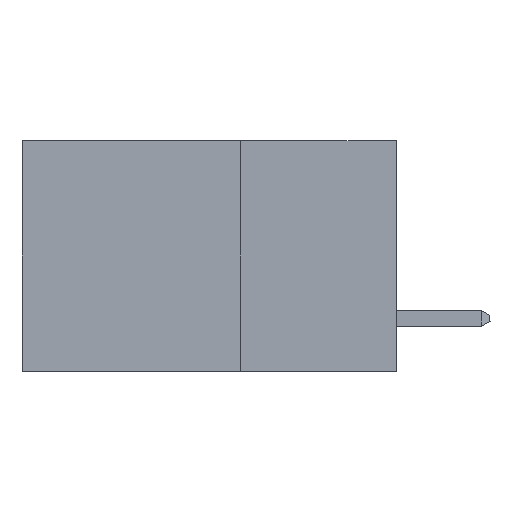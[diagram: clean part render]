
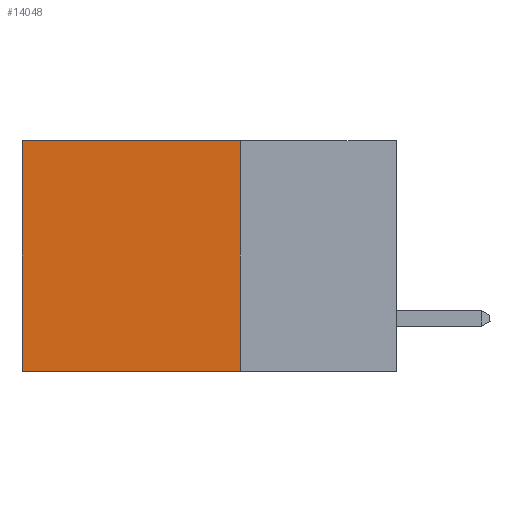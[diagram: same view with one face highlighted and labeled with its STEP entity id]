
A CAD part, left-side view. The second image highlights one B-rep face of the part: STEP entity #14048.
In plain terms, the highlighted planar face has unit normal (-1, 0, 0).
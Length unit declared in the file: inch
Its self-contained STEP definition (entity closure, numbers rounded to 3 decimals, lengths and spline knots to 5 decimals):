
#920 = DIRECTION ( 'NONE',  ( 0., 0., -1. ) ) ;
#1047 = DIRECTION ( 'NONE',  ( 0., 0., -1. ) ) ;
#1965 = VERTEX_POINT ( 'NONE', #13545 ) ;
#2149 = EDGE_LOOP ( 'NONE', ( #12952, #14968, #3069, #15810 ) ) ;
#2204 = FACE_OUTER_BOUND ( 'NONE', #2149, .T. ) ;
#2735 = LINE ( 'NONE', #10248, #9477 ) ;
#3069 = ORIENTED_EDGE ( 'NONE', *, *, #10551, .F. ) ;
#4941 = CARTESIAN_POINT ( 'NONE',  ( 0.298, 0.6, 0. ) ) ;
#5247 = DIRECTION ( 'NONE',  ( 0., 1., 0. ) ) ;
#5444 = EDGE_CURVE ( 'NONE', #1965, #18133, #12500, .T. ) ;
#5605 = CARTESIAN_POINT ( 'NONE',  ( 0.298, 0.6, -0.37 ) ) ;
#7328 = CARTESIAN_POINT ( 'NONE',  ( 0.298, 0.6, 0. ) ) ;
#7790 = DIRECTION ( 'NONE',  ( 1., 0., 0. ) ) ;
#9372 = DIRECTION ( 'NONE',  ( 0., 0., -1. ) ) ;
#9477 = VECTOR ( 'NONE', #5247, 39.37008 ) ;
#9799 = EDGE_CURVE ( 'NONE', #13871, #17910, #2735, .T. ) ;
#10248 = CARTESIAN_POINT ( 'NONE',  ( 0.298, 0.25, 0. ) ) ;
#10551 = EDGE_CURVE ( 'NONE', #13871, #1965, #19271, .T. ) ;
#12500 = LINE ( 'NONE', #14254, #20252 ) ;
#12952 = ORIENTED_EDGE ( 'NONE', *, *, #14503, .T. ) ;
#13545 = CARTESIAN_POINT ( 'NONE',  ( 0.298, 0.25, -0.37 ) ) ;
#13818 = VECTOR ( 'NONE', #1047, 39.37008 ) ;
#13871 = VERTEX_POINT ( 'NONE', #20360 ) ;
#14048 = ADVANCED_FACE ( 'NONE', ( #2204 ), #19338, .F. ) ;
#14254 = CARTESIAN_POINT ( 'NONE',  ( 0.298, 0.25, -0.37 ) ) ;
#14503 = EDGE_CURVE ( 'NONE', #17910, #18133, #15162, .T. ) ;
#14968 = ORIENTED_EDGE ( 'NONE', *, *, #5444, .F. ) ;
#15162 = LINE ( 'NONE', #7328, #20593 ) ;
#15810 = ORIENTED_EDGE ( 'NONE', *, *, #9799, .T. ) ;
#15920 = DIRECTION ( 'NONE',  ( 0., 1., 0. ) ) ;
#17482 = CARTESIAN_POINT ( 'NONE',  ( 0.298, 0.25, 0. ) ) ;
#17910 = VERTEX_POINT ( 'NONE', #4941 ) ;
#18133 = VERTEX_POINT ( 'NONE', #5605 ) ;
#19271 = LINE ( 'NONE', #17482, #13818 ) ;
#19338 = PLANE ( 'NONE',  #21119 ) ;
#19408 = CARTESIAN_POINT ( 'NONE',  ( 0.298, 0.25, 0. ) ) ;
#20252 = VECTOR ( 'NONE', #15920, 39.37008 ) ;
#20360 = CARTESIAN_POINT ( 'NONE',  ( 0.298, 0.25, 0. ) ) ;
#20593 = VECTOR ( 'NONE', #920, 39.37008 ) ;
#21119 = AXIS2_PLACEMENT_3D ( 'NONE', #19408, #7790, #9372 ) ;
